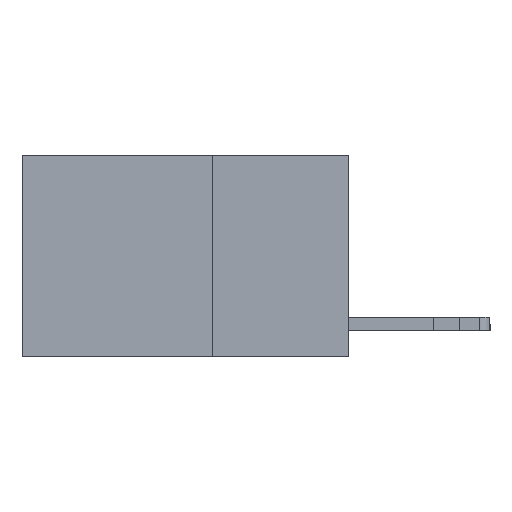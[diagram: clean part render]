
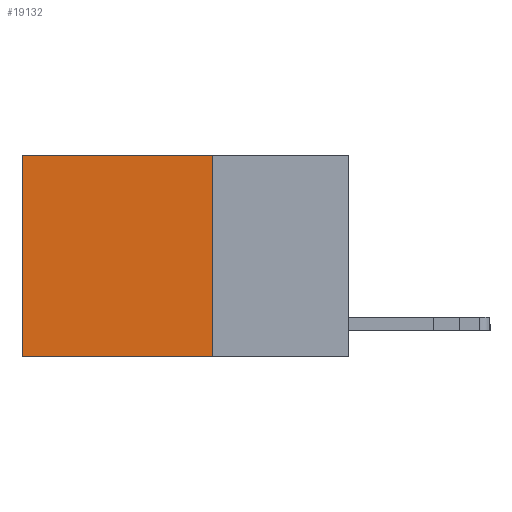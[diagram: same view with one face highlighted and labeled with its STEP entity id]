
A CAD part, left-side view. The second image highlights one B-rep face of the part: STEP entity #19132.
In plain terms, the highlighted planar face has unit normal (-1, 0, 0).
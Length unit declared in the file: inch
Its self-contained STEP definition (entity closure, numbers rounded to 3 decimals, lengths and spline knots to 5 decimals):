
#42 = LINE ( 'NONE', #13491, #15650 ) ;
#227 = EDGE_CURVE ( 'NONE', #7050, #3552, #1387, .T. ) ;
#1387 = LINE ( 'NONE', #5869, #17579 ) ;
#2357 = DIRECTION ( 'NONE',  ( 0., 0., -1. ) ) ;
#3382 = VERTEX_POINT ( 'NONE', #14569 ) ;
#3552 = VERTEX_POINT ( 'NONE', #18353 ) ;
#3559 = ORIENTED_EDGE ( 'NONE', *, *, #13274, .T. ) ;
#4646 = FACE_OUTER_BOUND ( 'NONE', #8184, .T. ) ;
#5385 = CARTESIAN_POINT ( 'NONE',  ( 0.2625, 0.25, -0.37 ) ) ;
#5588 = EDGE_CURVE ( 'NONE', #3552, #7772, #18490, .T. ) ;
#5869 = CARTESIAN_POINT ( 'NONE',  ( 0.2625, 0.25, 0. ) ) ;
#7050 = VERTEX_POINT ( 'NONE', #7191 ) ;
#7191 = CARTESIAN_POINT ( 'NONE',  ( 0.2625, 0.25, 0. ) ) ;
#7772 = VERTEX_POINT ( 'NONE', #9533 ) ;
#8017 = LINE ( 'NONE', #11519, #17971 ) ;
#8184 = EDGE_LOOP ( 'NONE', ( #3559, #8360, #17432, #19069 ) ) ;
#8360 = ORIENTED_EDGE ( 'NONE', *, *, #5588, .F. ) ;
#8441 = AXIS2_PLACEMENT_3D ( 'NONE', #15670, #12023, #18666 ) ;
#9533 = CARTESIAN_POINT ( 'NONE',  ( 0.2625, 0.6, -0.37 ) ) ;
#10136 = EDGE_CURVE ( 'NONE', #7050, #3382, #42, .T. ) ;
#11519 = CARTESIAN_POINT ( 'NONE',  ( 0.2625, 0.6, 0. ) ) ;
#12023 = DIRECTION ( 'NONE',  ( 1., 0., 0. ) ) ;
#12268 = DIRECTION ( 'NONE',  ( 0., 0., -1. ) ) ;
#13274 = EDGE_CURVE ( 'NONE', #3382, #7772, #8017, .T. ) ;
#13491 = CARTESIAN_POINT ( 'NONE',  ( 0.2625, 0.25, 0. ) ) ;
#13712 = PLANE ( 'NONE',  #8441 ) ;
#13972 = VECTOR ( 'NONE', #15495, 39.37008 ) ;
#14569 = CARTESIAN_POINT ( 'NONE',  ( 0.2625, 0.6, 0. ) ) ;
#15495 = DIRECTION ( 'NONE',  ( 0., 1., 0. ) ) ;
#15650 = VECTOR ( 'NONE', #19474, 39.37008 ) ;
#15670 = CARTESIAN_POINT ( 'NONE',  ( 0.2625, 0.25, 0. ) ) ;
#17432 = ORIENTED_EDGE ( 'NONE', *, *, #227, .F. ) ;
#17579 = VECTOR ( 'NONE', #12268, 39.37008 ) ;
#17971 = VECTOR ( 'NONE', #2357, 39.37008 ) ;
#18353 = CARTESIAN_POINT ( 'NONE',  ( 0.2625, 0.25, -0.37 ) ) ;
#18490 = LINE ( 'NONE', #5385, #13972 ) ;
#18666 = DIRECTION ( 'NONE',  ( 0., 0., -1. ) ) ;
#19069 = ORIENTED_EDGE ( 'NONE', *, *, #10136, .T. ) ;
#19132 = ADVANCED_FACE ( 'NONE', ( #4646 ), #13712, .F. ) ;
#19474 = DIRECTION ( 'NONE',  ( 0., 1., 0. ) ) ;
